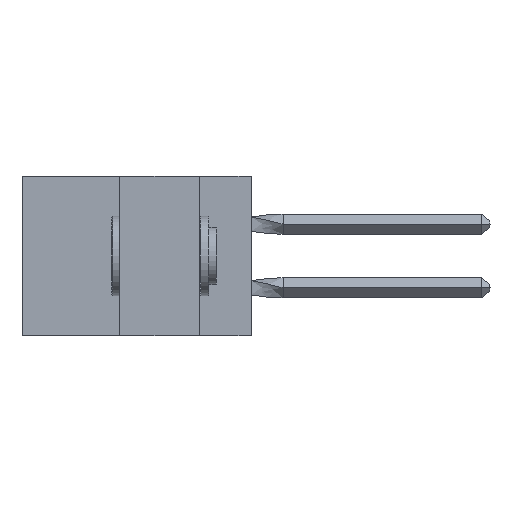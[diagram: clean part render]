
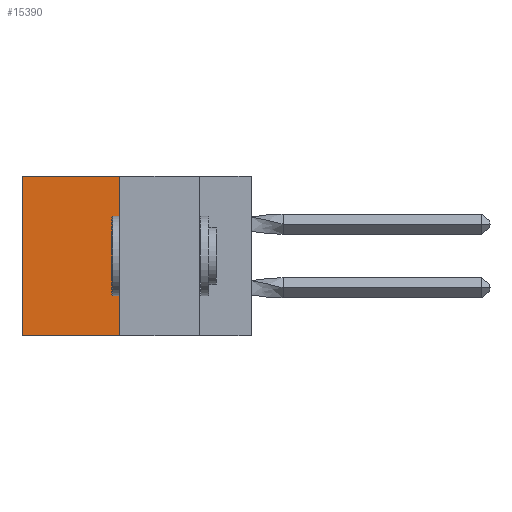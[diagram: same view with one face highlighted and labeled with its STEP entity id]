
A CAD part, left-side view. The second image highlights one B-rep face of the part: STEP entity #15390.
In plain terms, the highlighted planar face has unit normal (-1, 0, 0).
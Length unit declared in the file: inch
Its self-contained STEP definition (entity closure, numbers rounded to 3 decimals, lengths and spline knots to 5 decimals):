
#204 = DIRECTION ( 'NONE',  ( 0., 1., 0. ) ) ;
#751 = CARTESIAN_POINT ( 'NONE',  ( 0.305, 0.413, -0.5 ) ) ;
#977 = PLANE ( 'NONE',  #6059 ) ;
#1683 = EDGE_CURVE ( 'NONE', #5050, #10273, #6174, .T. ) ;
#2388 = CARTESIAN_POINT ( 'NONE',  ( 0.305, 0.72, 0. ) ) ;
#2766 = CARTESIAN_POINT ( 'NONE',  ( 0.305, 0.413, 0. ) ) ;
#4088 = DIRECTION ( 'NONE',  ( 0., 0., -1. ) ) ;
#4990 = VECTOR ( 'NONE', #204, 39.37008 ) ;
#5050 = VERTEX_POINT ( 'NONE', #14940 ) ;
#6052 = LINE ( 'NONE', #2766, #7678 ) ;
#6059 = AXIS2_PLACEMENT_3D ( 'NONE', #11475, #9898, #4088 ) ;
#6174 = LINE ( 'NONE', #13690, #4990 ) ;
#6358 = CARTESIAN_POINT ( 'NONE',  ( 0.305, 0.72, -0.5 ) ) ;
#7319 = CARTESIAN_POINT ( 'NONE',  ( 0.305, 0.72, -0.5 ) ) ;
#7678 = VECTOR ( 'NONE', #11715, 39.37008 ) ;
#7930 = CARTESIAN_POINT ( 'NONE',  ( 0.305, 0.413, 0. ) ) ;
#9898 = DIRECTION ( 'NONE',  ( 1., 0., 0. ) ) ;
#10273 = VERTEX_POINT ( 'NONE', #7319 ) ;
#10275 = ORIENTED_EDGE ( 'NONE', *, *, #1683, .F. ) ;
#10364 = EDGE_CURVE ( 'NONE', #11275, #11976, #6052, .T. ) ;
#10391 = ORIENTED_EDGE ( 'NONE', *, *, #16795, .F. ) ;
#11045 = ORIENTED_EDGE ( 'NONE', *, *, #10364, .T. ) ;
#11275 = VERTEX_POINT ( 'NONE', #7930 ) ;
#11319 = DIRECTION ( 'NONE',  ( 0., 0., -1. ) ) ;
#11475 = CARTESIAN_POINT ( 'NONE',  ( 0.305, 0.413, -0.5 ) ) ;
#11715 = DIRECTION ( 'NONE',  ( 0., 1., 0. ) ) ;
#11976 = VERTEX_POINT ( 'NONE', #2388 ) ;
#12057 = VECTOR ( 'NONE', #11319, 39.37008 ) ;
#12398 = VECTOR ( 'NONE', #12492, 39.37008 ) ;
#12492 = DIRECTION ( 'NONE',  ( 0., 0., -1. ) ) ;
#13690 = CARTESIAN_POINT ( 'NONE',  ( 0.305, 0.413, -0.5 ) ) ;
#14318 = EDGE_CURVE ( 'NONE', #11976, #10273, #19017, .T. ) ;
#14666 = LINE ( 'NONE', #751, #12057 ) ;
#14940 = CARTESIAN_POINT ( 'NONE',  ( 0.305, 0.413, -0.5 ) ) ;
#15390 = ADVANCED_FACE ( 'NONE', ( #18507 ), #977, .F. ) ;
#16368 = ORIENTED_EDGE ( 'NONE', *, *, #14318, .T. ) ;
#16795 = EDGE_CURVE ( 'NONE', #11275, #5050, #14666, .T. ) ;
#18507 = FACE_OUTER_BOUND ( 'NONE', #19130, .T. ) ;
#19017 = LINE ( 'NONE', #6358, #12398 ) ;
#19130 = EDGE_LOOP ( 'NONE', ( #16368, #10275, #10391, #11045 ) ) ;
